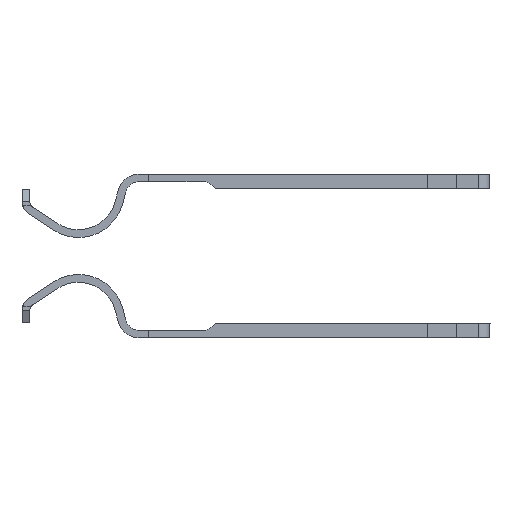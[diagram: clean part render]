
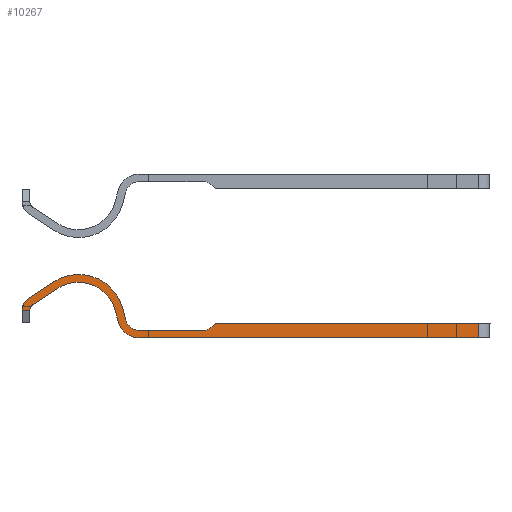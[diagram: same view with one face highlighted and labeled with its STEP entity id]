
A CAD part, left-side view. The second image highlights one B-rep face of the part: STEP entity #10267.
In plain terms, the highlighted face is planar.
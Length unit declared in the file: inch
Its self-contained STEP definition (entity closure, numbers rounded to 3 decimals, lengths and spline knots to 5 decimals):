
#343 = AXIS2_PLACEMENT_3D ( 'NONE', #25916, #25882, #25830 ) ;
#411 = CARTESIAN_POINT ( 'NONE',  ( 0.43721, 0.04723, 0.025 ) ) ;
#716 = VECTOR ( 'NONE', #7404, 39.37008 ) ;
#801 = VERTEX_POINT ( 'NONE', #15482 ) ;
#875 = LINE ( 'NONE', #7555, #716 ) ;
#993 = CARTESIAN_POINT ( 'NONE',  ( 0.28917, 0.05955, 0.025 ) ) ;
#1171 = ORIENTED_EDGE ( 'NONE', *, *, #19521, .F. ) ;
#1308 = DIRECTION ( 'NONE',  ( 1., 0., 0. ) ) ;
#1463 = EDGE_CURVE ( 'NONE', #17295, #1598, #23002, .T. ) ;
#1598 = VERTEX_POINT ( 'NONE', #20446 ) ;
#1686 = VECTOR ( 'NONE', #24406, 39.37008 ) ;
#1762 = CIRCLE ( 'NONE', #19849, 0.0135 ) ;
#1859 = CARTESIAN_POINT ( 'NONE',  ( 0.89821, 0.0375, 0.025 ) ) ;
#1866 = LINE ( 'NONE', #24586, #1686 ) ;
#1921 = CARTESIAN_POINT ( 'NONE',  ( 0.14621, 0.058, 0.025 ) ) ;
#2647 = CARTESIAN_POINT ( 'NONE',  ( 0.15971, 0.0575, 0.025 ) ) ;
#2769 = DIRECTION ( 'NONE',  ( 1., 0., 0. ) ) ;
#2801 = ORIENTED_EDGE ( 'NONE', *, *, #21257, .T. ) ;
#3557 = ORIENTED_EDGE ( 'NONE', *, *, #15980, .F. ) ;
#3591 = ORIENTED_EDGE ( 'NONE', *, *, #14136, .F. ) ;
#3880 = ORIENTED_EDGE ( 'NONE', *, *, #19801, .T. ) ;
#3998 = VECTOR ( 'NONE', #14161, 39.37008 ) ;
#4235 = VECTOR ( 'NONE', #7572, 39.37008 ) ;
#4262 = LINE ( 'NONE', #16058, #4235 ) ;
#4274 = ORIENTED_EDGE ( 'NONE', *, *, #12721, .T. ) ;
#4411 = LINE ( 'NONE', #18265, #3998 ) ;
#4541 = FACE_OUTER_BOUND ( 'NONE', #16147, .T. ) ;
#4850 = DIRECTION ( 'NONE',  ( -1., 0., 0. ) ) ;
#5409 = VERTEX_POINT ( 'NONE', #27169 ) ;
#5423 = CARTESIAN_POINT ( 'NONE',  ( 0.19317, 0.09559, 0.025 ) ) ;
#6072 = AXIS2_PLACEMENT_3D ( 'NONE', #411, #15707, #2769 ) ;
#6190 = VERTEX_POINT ( 'NONE', #18134 ) ;
#6308 = DIRECTION ( 'NONE',  ( 0., 0., 1. ) ) ;
#6448 = VERTEX_POINT ( 'NONE', #11801 ) ;
#6622 = EDGE_CURVE ( 'NONE', #6448, #25252, #875, .T. ) ;
#7097 = VERTEX_POINT ( 'NONE', #19934 ) ;
#7404 = DIRECTION ( 'NONE',  ( 1., 0., 0. ) ) ;
#7555 = CARTESIAN_POINT ( 'NONE',  ( 0.33, 0.0255, 0.025 ) ) ;
#7572 = DIRECTION ( 'NONE',  ( -0.707, -0.707, 0. ) ) ;
#7647 = VECTOR ( 'NONE', #26926, 39.37008 ) ;
#7734 = DIRECTION ( 'NONE',  ( -1., 0., 0. ) ) ;
#7826 = DIRECTION ( 'NONE',  ( 0., 0., -1. ) ) ;
#8065 = DIRECTION ( 'NONE',  ( 0., 0., -1. ) ) ;
#8142 = LINE ( 'NONE', #993, #7647 ) ;
#8396 = PLANE ( 'NONE',  #26202 ) ;
#8852 = CARTESIAN_POINT ( 'NONE',  ( 0.43721, 0.0255, 0.025 ) ) ;
#9521 = AXIS2_PLACEMENT_3D ( 'NONE', #18999, #6308, #21071 ) ;
#9568 = EDGE_CURVE ( 'NONE', #24475, #16167, #12334, .T. ) ;
#9798 = CARTESIAN_POINT ( 'NONE',  ( 0.89821, 0.0125, 0.025 ) ) ;
#10170 = CARTESIAN_POINT ( 'NONE',  ( 0.13322, 0.058, 0.025 ) ) ;
#10267 = ADVANCED_FACE ( 'NONE', ( #4541 ), #8396, .F. ) ;
#10367 = DIRECTION ( 'NONE',  ( 1., 0., 0. ) ) ;
#10421 = VERTEX_POINT ( 'NONE', #24895 ) ;
#10434 = DIRECTION ( 'NONE',  ( 0., 0., 1. ) ) ;
#10459 = CARTESIAN_POINT ( 'NONE',  ( 0.33, 0.049, 0.025 ) ) ;
#11128 = EDGE_CURVE ( 'NONE', #13716, #27328, #24768, .T. ) ;
#11522 = CARTESIAN_POINT ( 'NONE',  ( 0.095, 0.025, 0.025 ) ) ;
#11801 = CARTESIAN_POINT ( 'NONE',  ( 0.33, 0.0255, 0.025 ) ) ;
#12149 = EDGE_CURVE ( 'NONE', #16406, #10421, #17059, .T. ) ;
#12334 = CIRCLE ( 'NONE', #18983, 0.0765 ) ;
#12721 = EDGE_CURVE ( 'NONE', #13716, #801, #13169, .T. ) ;
#12740 = VECTOR ( 'NONE', #14975, 39.37008 ) ;
#12787 = ORIENTED_EDGE ( 'NONE', *, *, #6622, .F. ) ;
#12870 = LINE ( 'NONE', #27221, #12740 ) ;
#13169 = LINE ( 'NONE', #1921, #13240 ) ;
#13240 = VECTOR ( 'NONE', #1308, 39.37008 ) ;
#13352 = EDGE_CURVE ( 'NONE', #6190, #16406, #8142, .T. ) ;
#13377 = CARTESIAN_POINT ( 'NONE',  ( 0.30169, 0.06304, 0.025 ) ) ;
#13552 = DIRECTION ( 'NONE',  ( -1., 0., 0. ) ) ;
#13708 = DIRECTION ( 'NONE',  ( 0., 0., -1. ) ) ;
#13716 = VERTEX_POINT ( 'NONE', #10170 ) ;
#13733 = CARTESIAN_POINT ( 'NONE',  ( 0.228, 0.0425, 0.025 ) ) ;
#14136 = EDGE_CURVE ( 'NONE', #16167, #5409, #1866, .T. ) ;
#14161 = DIRECTION ( 'NONE',  ( 0.836, 0.549, 0. ) ) ;
#14308 = CIRCLE ( 'NONE', #16405, 0.0635 ) ;
#14975 = DIRECTION ( 'NONE',  ( 0., -1., 0. ) ) ;
#15482 = CARTESIAN_POINT ( 'NONE',  ( 0.14622, 0.058, 0.025 ) ) ;
#15707 = DIRECTION ( 'NONE',  ( 0., 0., -1. ) ) ;
#15844 = VECTOR ( 'NONE', #17454, 39.37008 ) ;
#15943 = ORIENTED_EDGE ( 'NONE', *, *, #24853, .T. ) ;
#15980 = EDGE_CURVE ( 'NONE', #17295, #18253, #12870, .T. ) ;
#16058 = CARTESIAN_POINT ( 'NONE',  ( 0.45821, 0.0375, 0.025 ) ) ;
#16066 = LINE ( 'NONE', #19518, #15844 ) ;
#16147 = EDGE_LOOP ( 'NONE', ( #21026, #4274, #20739, #2801, #19182, #20810, #22621, #3880, #3557, #19147, #19707, #15943, #12787, #19780, #3591, #18256, #1171 ) ) ;
#16167 = VERTEX_POINT ( 'NONE', #13377 ) ;
#16405 = AXIS2_PLACEMENT_3D ( 'NONE', #20436, #7826, #22454 ) ;
#16406 = VERTEX_POINT ( 'NONE', #24431 ) ;
#17059 = CIRCLE ( 'NONE', #18125, 0.0365 ) ;
#17250 = CIRCLE ( 'NONE', #9521, 0.0235 ) ;
#17295 = VERTEX_POINT ( 'NONE', #1859 ) ;
#17454 = DIRECTION ( 'NONE',  ( 1., 0., 0. ) ) ;
#17629 = DIRECTION ( 'NONE',  ( 0., 0., -1. ) ) ;
#17721 = LINE ( 'NONE', #22744, #17746 ) ;
#17746 = VECTOR ( 'NONE', #24827, 39.37008 ) ;
#18125 = AXIS2_PLACEMENT_3D ( 'NONE', #10459, #10434, #10367 ) ;
#18134 = CARTESIAN_POINT ( 'NONE',  ( 0.28917, 0.05955, 0.025 ) ) ;
#18231 = CARTESIAN_POINT ( 'NONE',  ( 0.15231, 0.06879, 0.025 ) ) ;
#18253 = VERTEX_POINT ( 'NONE', #9798 ) ;
#18256 = ORIENTED_EDGE ( 'NONE', *, *, #9568, .F. ) ;
#18265 = CARTESIAN_POINT ( 'NONE',  ( 0.15231, 0.06879, 0.025 ) ) ;
#18983 = AXIS2_PLACEMENT_3D ( 'NONE', #13733, #13708, #13552 ) ;
#18999 = CARTESIAN_POINT ( 'NONE',  ( 0.33, 0.049, 0.025 ) ) ;
#19147 = ORIENTED_EDGE ( 'NONE', *, *, #1463, .T. ) ;
#19182 = ORIENTED_EDGE ( 'NONE', *, *, #20097, .T. ) ;
#19518 = CARTESIAN_POINT ( 'NONE',  ( 0.33, 0.0125, 0.025 ) ) ;
#19521 = EDGE_CURVE ( 'NONE', #27328, #24475, #17721, .T. ) ;
#19529 = CARTESIAN_POINT ( 'NONE',  ( 0.14518, 0.07966, 0.025 ) ) ;
#19613 = EDGE_CURVE ( 'NONE', #5409, #6448, #17250, .T. ) ;
#19707 = ORIENTED_EDGE ( 'NONE', *, *, #21198, .T. ) ;
#19780 = ORIENTED_EDGE ( 'NONE', *, *, #19613, .F. ) ;
#19801 = EDGE_CURVE ( 'NONE', #10421, #18253, #16066, .T. ) ;
#19849 = AXIS2_PLACEMENT_3D ( 'NONE', #2647, #17629, #4850 ) ;
#19934 = CARTESIAN_POINT ( 'NONE',  ( 0.45258, 0.03186, 0.025 ) ) ;
#20071 = VERTEX_POINT ( 'NONE', #18231 ) ;
#20097 = EDGE_CURVE ( 'NONE', #23691, #6190, #14308, .T. ) ;
#20418 = CARTESIAN_POINT ( 'NONE',  ( 0.18604, 0.10646, 0.025 ) ) ;
#20436 = CARTESIAN_POINT ( 'NONE',  ( 0.228, 0.0425, 0.025 ) ) ;
#20446 = CARTESIAN_POINT ( 'NONE',  ( 0.45821, 0.0375, 0.025 ) ) ;
#20739 = ORIENTED_EDGE ( 'NONE', *, *, #21565, .T. ) ;
#20810 = ORIENTED_EDGE ( 'NONE', *, *, #13352, .T. ) ;
#21026 = ORIENTED_EDGE ( 'NONE', *, *, #11128, .F. ) ;
#21071 = DIRECTION ( 'NONE',  ( 1., 0., 0. ) ) ;
#21198 = EDGE_CURVE ( 'NONE', #1598, #7097, #4262, .T. ) ;
#21257 = EDGE_CURVE ( 'NONE', #20071, #23691, #4411, .T. ) ;
#21565 = EDGE_CURVE ( 'NONE', #801, #20071, #1762, .T. ) ;
#22372 = CARTESIAN_POINT ( 'NONE',  ( 0.45821, 0.0375, 0.025 ) ) ;
#22454 = DIRECTION ( 'NONE',  ( -1., 0., 0. ) ) ;
#22490 = DIRECTION ( 'NONE',  ( -1., 0., 0. ) ) ;
#22621 = ORIENTED_EDGE ( 'NONE', *, *, #12149, .T. ) ;
#22744 = CARTESIAN_POINT ( 'NONE',  ( 0.14518, 0.07966, 0.025 ) ) ;
#22927 = VECTOR ( 'NONE', #22490, 39.37008 ) ;
#23002 = LINE ( 'NONE', #22372, #22927 ) ;
#23691 = VERTEX_POINT ( 'NONE', #5423 ) ;
#24086 = CIRCLE ( 'NONE', #6072, 0.02173 ) ;
#24406 = DIRECTION ( 'NONE',  ( 0.268, -0.963, 0. ) ) ;
#24431 = CARTESIAN_POINT ( 'NONE',  ( 0.29484, 0.0392, 0.025 ) ) ;
#24475 = VERTEX_POINT ( 'NONE', #20418 ) ;
#24586 = CARTESIAN_POINT ( 'NONE',  ( 0.30169, 0.06304, 0.025 ) ) ;
#24768 = CIRCLE ( 'NONE', #343, 0.0265 ) ;
#24827 = DIRECTION ( 'NONE',  ( 0.836, 0.549, 0. ) ) ;
#24853 = EDGE_CURVE ( 'NONE', #7097, #25252, #24086, .T. ) ;
#24895 = CARTESIAN_POINT ( 'NONE',  ( 0.33, 0.0125, 0.025 ) ) ;
#25252 = VERTEX_POINT ( 'NONE', #8852 ) ;
#25830 = DIRECTION ( 'NONE',  ( -1., 0., 0. ) ) ;
#25882 = DIRECTION ( 'NONE',  ( 0., 0., -1. ) ) ;
#25916 = CARTESIAN_POINT ( 'NONE',  ( 0.15971, 0.0575, 0.025 ) ) ;
#26202 = AXIS2_PLACEMENT_3D ( 'NONE', #11522, #8065, #7734 ) ;
#26926 = DIRECTION ( 'NONE',  ( 0.268, -0.963, 0. ) ) ;
#27169 = CARTESIAN_POINT ( 'NONE',  ( 0.30736, 0.04269, 0.025 ) ) ;
#27221 = CARTESIAN_POINT ( 'NONE',  ( 0.89821, 0.37918, 0.025 ) ) ;
#27328 = VERTEX_POINT ( 'NONE', #19529 ) ;
